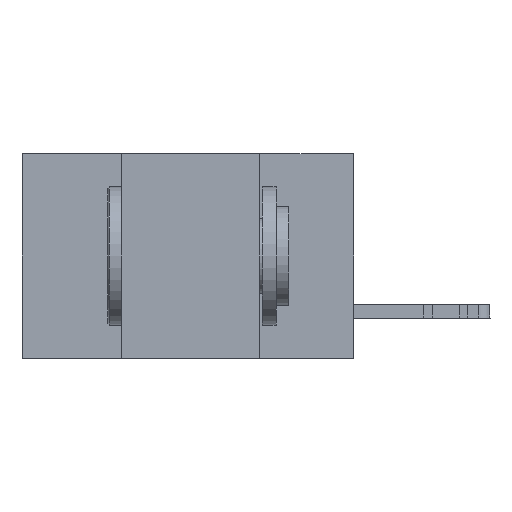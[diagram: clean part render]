
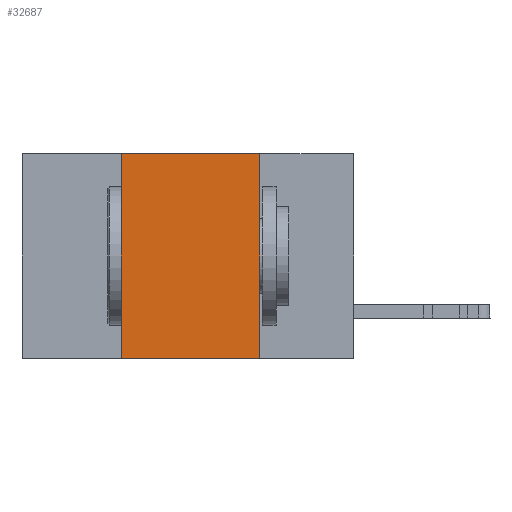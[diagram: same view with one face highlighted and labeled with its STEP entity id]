
A CAD part, left-side view. The second image highlights one B-rep face of the part: STEP entity #32687.
In plain terms, the highlighted planar face has unit normal (-1, 0, 0).
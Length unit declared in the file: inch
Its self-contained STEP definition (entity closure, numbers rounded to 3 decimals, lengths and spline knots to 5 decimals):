
#142 = PLANE ( 'NONE',  #40056 ) ;
#2202 = CARTESIAN_POINT ( 'NONE',  ( 0., 0.42, -0.37 ) ) ;
#2625 = VERTEX_POINT ( 'NONE', #27006 ) ;
#3326 = DIRECTION ( 'NONE',  ( 0., 0., -1. ) ) ;
#3719 = VERTEX_POINT ( 'NONE', #4892 ) ;
#4892 = CARTESIAN_POINT ( 'NONE',  ( 0., 0.42, 0. ) ) ;
#6559 = EDGE_CURVE ( 'NONE', #16045, #3719, #32892, .T. ) ;
#6633 = CARTESIAN_POINT ( 'NONE',  ( 0., 0.42, 0. ) ) ;
#7407 = EDGE_CURVE ( 'NONE', #33599, #2625, #36343, .T. ) ;
#8852 = EDGE_CURVE ( 'NONE', #3719, #33599, #19229, .T. ) ;
#10254 = EDGE_CURVE ( 'NONE', #16045, #2625, #26169, .T. ) ;
#10553 = DIRECTION ( 'NONE',  ( 0., -1., 0. ) ) ;
#12426 = CARTESIAN_POINT ( 'NONE',  ( 0., 0.6, -0.37 ) ) ;
#13228 = EDGE_LOOP ( 'NONE', ( #26055, #37517, #22658, #32706 ) ) ;
#16045 = VERTEX_POINT ( 'NONE', #2202 ) ;
#19229 = LINE ( 'NONE', #30088, #31782 ) ;
#22333 = DIRECTION ( 'NONE',  ( 1., 0., 0. ) ) ;
#22603 = CARTESIAN_POINT ( 'NONE',  ( 0., 0.6, 0. ) ) ;
#22658 = ORIENTED_EDGE ( 'NONE', *, *, #6559, .F. ) ;
#24514 = CARTESIAN_POINT ( 'NONE',  ( 0., 0.17, 0. ) ) ;
#24986 = FACE_OUTER_BOUND ( 'NONE', #13228, .T. ) ;
#26055 = ORIENTED_EDGE ( 'NONE', *, *, #7407, .F. ) ;
#26169 = LINE ( 'NONE', #12426, #32184 ) ;
#27006 = CARTESIAN_POINT ( 'NONE',  ( 0., 0.17, -0.37 ) ) ;
#27157 = DIRECTION ( 'NONE',  ( 0., -1., 0. ) ) ;
#30088 = CARTESIAN_POINT ( 'NONE',  ( 0., 0.6, 0. ) ) ;
#31077 = DIRECTION ( 'NONE',  ( 0., 0., 1. ) ) ;
#31782 = VECTOR ( 'NONE', #27157, 39.37008 ) ;
#32184 = VECTOR ( 'NONE', #10553, 39.37008 ) ;
#32687 = ADVANCED_FACE ( 'NONE', ( #24986 ), #142, .F. ) ;
#32706 = ORIENTED_EDGE ( 'NONE', *, *, #10254, .T. ) ;
#32892 = LINE ( 'NONE', #6633, #39445 ) ;
#33163 = CARTESIAN_POINT ( 'NONE',  ( 0., 0.17, 0. ) ) ;
#33599 = VERTEX_POINT ( 'NONE', #33163 ) ;
#36343 = LINE ( 'NONE', #24514, #39866 ) ;
#37517 = ORIENTED_EDGE ( 'NONE', *, *, #8852, .F. ) ;
#38590 = DIRECTION ( 'NONE',  ( 0., 0., -1. ) ) ;
#39445 = VECTOR ( 'NONE', #31077, 39.37008 ) ;
#39866 = VECTOR ( 'NONE', #3326, 39.37008 ) ;
#40056 = AXIS2_PLACEMENT_3D ( 'NONE', #22603, #22333, #38590 ) ;
